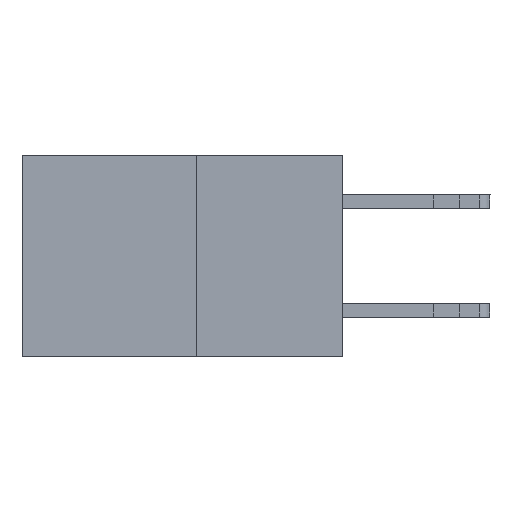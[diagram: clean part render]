
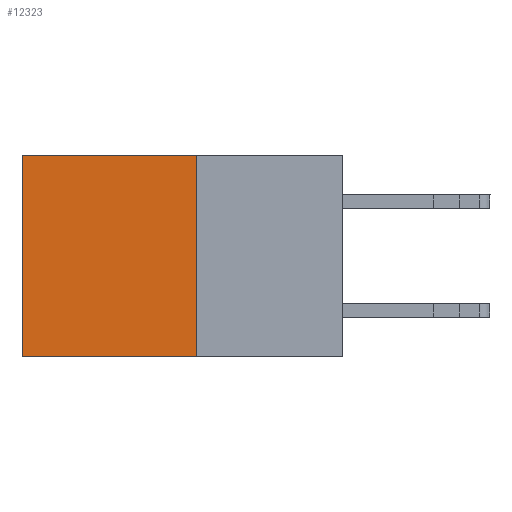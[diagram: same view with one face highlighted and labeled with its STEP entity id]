
A CAD part, left-side view. The second image highlights one B-rep face of the part: STEP entity #12323.
In plain terms, the highlighted planar face has unit normal (-1, 0, 0).
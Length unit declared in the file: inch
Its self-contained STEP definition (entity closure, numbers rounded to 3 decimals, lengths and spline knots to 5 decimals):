
#260 = VECTOR ( 'NONE', #18835, 39.37008 ) ;
#863 = VERTEX_POINT ( 'NONE', #13690 ) ;
#1392 = DIRECTION ( 'NONE',  ( 0., 1., 0. ) ) ;
#1819 = CARTESIAN_POINT ( 'NONE',  ( 0.277, 0.27, 0. ) ) ;
#3006 = EDGE_CURVE ( 'NONE', #24379, #863, #7151, .T. ) ;
#3402 = VERTEX_POINT ( 'NONE', #21749 ) ;
#4084 = ORIENTED_EDGE ( 'NONE', *, *, #3006, .T. ) ;
#5214 = LINE ( 'NONE', #23502, #7799 ) ;
#7151 = LINE ( 'NONE', #17735, #11599 ) ;
#7799 = VECTOR ( 'NONE', #24295, 39.37008 ) ;
#7827 = CARTESIAN_POINT ( 'NONE',  ( 0.277, 0.27, 0. ) ) ;
#8401 = CARTESIAN_POINT ( 'NONE',  ( 0.277, 0.27, -0.37 ) ) ;
#10475 = AXIS2_PLACEMENT_3D ( 'NONE', #22013, #26188, #17406 ) ;
#11599 = VECTOR ( 'NONE', #15217, 39.37008 ) ;
#12323 = ADVANCED_FACE ( 'NONE', ( #25902 ), #17698, .F. ) ;
#12526 = LINE ( 'NONE', #7827, #16135 ) ;
#12727 = ORIENTED_EDGE ( 'NONE', *, *, #13256, .F. ) ;
#13256 = EDGE_CURVE ( 'NONE', #3402, #863, #5214, .T. ) ;
#13394 = EDGE_CURVE ( 'NONE', #23379, #3402, #25111, .T. ) ;
#13690 = CARTESIAN_POINT ( 'NONE',  ( 0.277, 0.59, -0.37 ) ) ;
#15217 = DIRECTION ( 'NONE',  ( 0., 0., -1. ) ) ;
#16135 = VECTOR ( 'NONE', #1392, 39.37008 ) ;
#17311 = EDGE_LOOP ( 'NONE', ( #4084, #12727, #18568, #24019 ) ) ;
#17406 = DIRECTION ( 'NONE',  ( 0., 0., -1. ) ) ;
#17698 = PLANE ( 'NONE',  #10475 ) ;
#17735 = CARTESIAN_POINT ( 'NONE',  ( 0.277, 0.59, -0.37 ) ) ;
#18568 = ORIENTED_EDGE ( 'NONE', *, *, #13394, .F. ) ;
#18835 = DIRECTION ( 'NONE',  ( 0., 0., -1. ) ) ;
#18876 = CARTESIAN_POINT ( 'NONE',  ( 0.277, 0.59, 0. ) ) ;
#21749 = CARTESIAN_POINT ( 'NONE',  ( 0.277, 0.27, -0.37 ) ) ;
#22013 = CARTESIAN_POINT ( 'NONE',  ( 0.277, 0.27, -0.37 ) ) ;
#23379 = VERTEX_POINT ( 'NONE', #1819 ) ;
#23502 = CARTESIAN_POINT ( 'NONE',  ( 0.277, 0.27, -0.37 ) ) ;
#24019 = ORIENTED_EDGE ( 'NONE', *, *, #26814, .T. ) ;
#24295 = DIRECTION ( 'NONE',  ( 0., 1., 0. ) ) ;
#24379 = VERTEX_POINT ( 'NONE', #18876 ) ;
#25111 = LINE ( 'NONE', #8401, #260 ) ;
#25902 = FACE_OUTER_BOUND ( 'NONE', #17311, .T. ) ;
#26188 = DIRECTION ( 'NONE',  ( 1., 0., 0. ) ) ;
#26814 = EDGE_CURVE ( 'NONE', #23379, #24379, #12526, .T. ) ;
